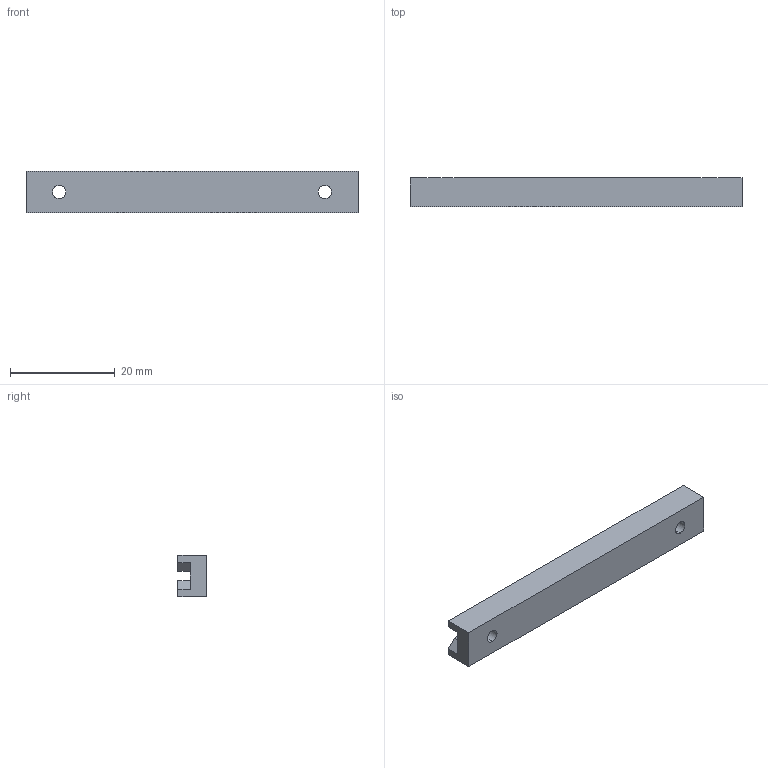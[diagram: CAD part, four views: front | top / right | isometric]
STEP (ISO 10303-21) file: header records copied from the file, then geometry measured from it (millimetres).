
FILE_DESCRIPTION (( 'STEP AP214' ), '1' );
FILE_NAME ('616-220-302.STEP', '2020-08-20T18:08:17', ( '' ), ( '' ), 'SwSTEP 2.0', 'SolidWorks 2020', '' );
FILE_SCHEMA (( 'AUTOMOTIVE_DESIGN' ));
Length unit declared in the file: inch
Products named in the file (1): 616-220-302
Bounding box: 63.5 x 5.66 x 7.92 mm (x, y, z)
Volume: 2399 mm3; surface area: 2150.7 mm2
Topology: 1 solids, 1 shells, 284 faces, 753 edges, 502 vertices
Faces by surface type: plane 176, bspline 100, cylinder 8
Entity records: 14777 total; most frequent: CARTESIAN_POINT 8328, ORIENTED_EDGE 1506, DIRECTION 947, EDGE_CURVE 753, LINE 529, VECTOR 529, VERTEX_POINT 502, EDGE_LOOP 319
